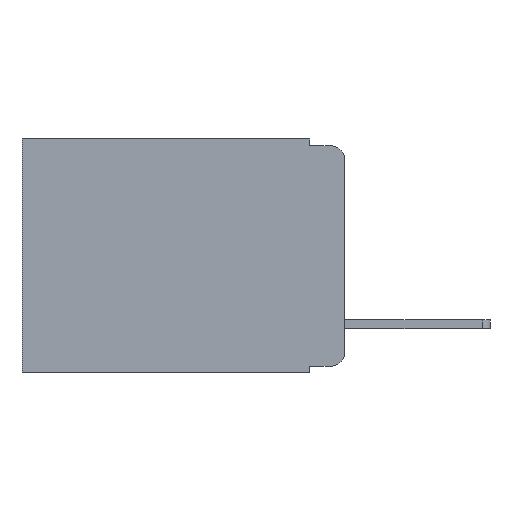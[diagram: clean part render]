
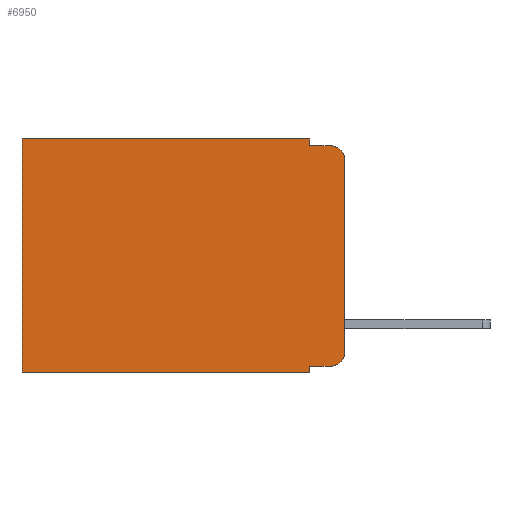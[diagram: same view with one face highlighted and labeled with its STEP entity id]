
A CAD part, left-side view. The second image highlights one B-rep face of the part: STEP entity #6950.
In plain terms, the highlighted planar face has unit normal (-1, 0, 0).
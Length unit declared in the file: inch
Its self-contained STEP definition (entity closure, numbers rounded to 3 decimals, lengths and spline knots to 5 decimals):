
#126 = ORIENTED_EDGE ( 'NONE', *, *, #15734, .T. ) ;
#668 = ORIENTED_EDGE ( 'NONE', *, *, #15099, .F. ) ;
#844 = LINE ( 'NONE', #11927, #1366 ) ;
#855 = CARTESIAN_POINT ( 'NONE',  ( 0.298, 0., -0.343 ) ) ;
#1202 = CARTESIAN_POINT ( 'NONE',  ( 0.298, 0., -0.313 ) ) ;
#1366 = VECTOR ( 'NONE', #3094, 39.37008 ) ;
#1483 = CARTESIAN_POINT ( 'NONE',  ( 0.298, 0.473, -0.343 ) ) ;
#1614 = DIRECTION ( 'NONE',  ( -1., 0., 0. ) ) ;
#1718 = ORIENTED_EDGE ( 'NONE', *, *, #3672, .T. ) ;
#1752 = CARTESIAN_POINT ( 'NONE',  ( 0.298, 0.051, -0.333 ) ) ;
#1792 = CARTESIAN_POINT ( 'NONE',  ( 0.298, 0.051, -0.01 ) ) ;
#1879 = CARTESIAN_POINT ( 'NONE',  ( 0.298, 0.051, 0. ) ) ;
#1960 = VECTOR ( 'NONE', #5044, 39.37008 ) ;
#1992 = EDGE_CURVE ( 'NONE', #5318, #4289, #844, .T. ) ;
#2191 = VERTEX_POINT ( 'NONE', #1752 ) ;
#2239 = FACE_OUTER_BOUND ( 'NONE', #7586, .T. ) ;
#2647 = VECTOR ( 'NONE', #3571, 39.37008 ) ;
#2851 = VECTOR ( 'NONE', #9637, 39.37008 ) ;
#3016 = ORIENTED_EDGE ( 'NONE', *, *, #11231, .F. ) ;
#3094 = DIRECTION ( 'NONE',  ( 0., 1., 0. ) ) ;
#3420 = DIRECTION ( 'NONE',  ( 0., -1., 0. ) ) ;
#3571 = DIRECTION ( 'NONE',  ( 0., 0., -1. ) ) ;
#3672 = EDGE_CURVE ( 'NONE', #4289, #11969, #14026, .T. ) ;
#4289 = VERTEX_POINT ( 'NONE', #9174 ) ;
#4348 = CIRCLE ( 'NONE', #9840, 0.02 ) ;
#4372 = VERTEX_POINT ( 'NONE', #16258 ) ;
#4491 = CARTESIAN_POINT ( 'NONE',  ( 0.298, 0.051, -0.01 ) ) ;
#4527 = ORIENTED_EDGE ( 'NONE', *, *, #7503, .T. ) ;
#4636 = PLANE ( 'NONE',  #16531 ) ;
#4700 = EDGE_CURVE ( 'NONE', #12864, #11802, #14371, .T. ) ;
#4959 = AXIS2_PLACEMENT_3D ( 'NONE', #6357, #15957, #7825 ) ;
#4982 = EDGE_CURVE ( 'NONE', #11030, #11802, #4348, .T. ) ;
#5044 = DIRECTION ( 'NONE',  ( 0., 0., -1. ) ) ;
#5260 = LINE ( 'NONE', #855, #15924 ) ;
#5318 = VERTEX_POINT ( 'NONE', #7589 ) ;
#6235 = DIRECTION ( 'NONE',  ( 1., 0., 0. ) ) ;
#6240 = LINE ( 'NONE', #9405, #1960 ) ;
#6357 = CARTESIAN_POINT ( 'NONE',  ( 0.298, 0.02, -0.03 ) ) ;
#6654 = VECTOR ( 'NONE', #11304, 39.37008 ) ;
#6688 = EDGE_CURVE ( 'NONE', #13576, #11969, #5260, .T. ) ;
#6950 = ADVANCED_FACE ( 'NONE', ( #2239 ), #4636, .F. ) ;
#7163 = ORIENTED_EDGE ( 'NONE', *, *, #1992, .T. ) ;
#7261 = DIRECTION ( 'NONE',  ( 0., 1., 0. ) ) ;
#7503 = EDGE_CURVE ( 'NONE', #2191, #11030, #13018, .T. ) ;
#7517 = CARTESIAN_POINT ( 'NONE',  ( 0.298, 0.051, -0.343 ) ) ;
#7586 = EDGE_LOOP ( 'NONE', ( #7627, #126, #3016, #17576, #7163, #1718, #16565, #668, #4527, #8962 ) ) ;
#7589 = CARTESIAN_POINT ( 'NONE',  ( 0.298, 0.051, 0. ) ) ;
#7627 = ORIENTED_EDGE ( 'NONE', *, *, #4700, .F. ) ;
#7825 = DIRECTION ( 'NONE',  ( 0., 0., -1. ) ) ;
#8247 = CARTESIAN_POINT ( 'NONE',  ( 0.298, 0., 0. ) ) ;
#8799 = CARTESIAN_POINT ( 'NONE',  ( 0.298, 0.051, -0.333 ) ) ;
#8930 = VECTOR ( 'NONE', #16871, 39.37008 ) ;
#8962 = ORIENTED_EDGE ( 'NONE', *, *, #4982, .T. ) ;
#9174 = CARTESIAN_POINT ( 'NONE',  ( 0.298, 0.473, 0. ) ) ;
#9405 = CARTESIAN_POINT ( 'NONE',  ( 0.298, 0.051, 0. ) ) ;
#9637 = DIRECTION ( 'NONE',  ( 0., 0., -1. ) ) ;
#9687 = CIRCLE ( 'NONE', #4959, 0.02 ) ;
#9840 = AXIS2_PLACEMENT_3D ( 'NONE', #10635, #1614, #12037 ) ;
#9859 = VERTEX_POINT ( 'NONE', #4491 ) ;
#9860 = CARTESIAN_POINT ( 'NONE',  ( 0.298, 0.473, 0. ) ) ;
#10511 = CARTESIAN_POINT ( 'NONE',  ( 0.298, 0., -0.03 ) ) ;
#10552 = LINE ( 'NONE', #1879, #2647 ) ;
#10635 = CARTESIAN_POINT ( 'NONE',  ( 0.298, 0.02, -0.313 ) ) ;
#11030 = VERTEX_POINT ( 'NONE', #17130 ) ;
#11231 = EDGE_CURVE ( 'NONE', #9859, #4372, #12632, .T. ) ;
#11304 = DIRECTION ( 'NONE',  ( 0., 0., -1. ) ) ;
#11802 = VERTEX_POINT ( 'NONE', #1202 ) ;
#11927 = CARTESIAN_POINT ( 'NONE',  ( 0.298, 0., 0. ) ) ;
#11969 = VERTEX_POINT ( 'NONE', #1483 ) ;
#12037 = DIRECTION ( 'NONE',  ( 0., 0., -1. ) ) ;
#12168 = EDGE_CURVE ( 'NONE', #5318, #9859, #6240, .T. ) ;
#12632 = LINE ( 'NONE', #1792, #16149 ) ;
#12864 = VERTEX_POINT ( 'NONE', #10511 ) ;
#13018 = LINE ( 'NONE', #8799, #8930 ) ;
#13576 = VERTEX_POINT ( 'NONE', #7517 ) ;
#14026 = LINE ( 'NONE', #9860, #6654 ) ;
#14371 = LINE ( 'NONE', #8247, #2851 ) ;
#14540 = CARTESIAN_POINT ( 'NONE',  ( 0.298, 0., 0. ) ) ;
#15099 = EDGE_CURVE ( 'NONE', #2191, #13576, #10552, .T. ) ;
#15734 = EDGE_CURVE ( 'NONE', #12864, #4372, #9687, .T. ) ;
#15850 = DIRECTION ( 'NONE',  ( 0., 0., -1. ) ) ;
#15924 = VECTOR ( 'NONE', #7261, 39.37008 ) ;
#15957 = DIRECTION ( 'NONE',  ( -1., 0., 0. ) ) ;
#16149 = VECTOR ( 'NONE', #3420, 39.37008 ) ;
#16258 = CARTESIAN_POINT ( 'NONE',  ( 0.298, 0.02, -0.01 ) ) ;
#16531 = AXIS2_PLACEMENT_3D ( 'NONE', #14540, #6235, #15850 ) ;
#16565 = ORIENTED_EDGE ( 'NONE', *, *, #6688, .F. ) ;
#16871 = DIRECTION ( 'NONE',  ( 0., -1., 0. ) ) ;
#17130 = CARTESIAN_POINT ( 'NONE',  ( 0.298, 0.02, -0.333 ) ) ;
#17576 = ORIENTED_EDGE ( 'NONE', *, *, #12168, .F. ) ;
